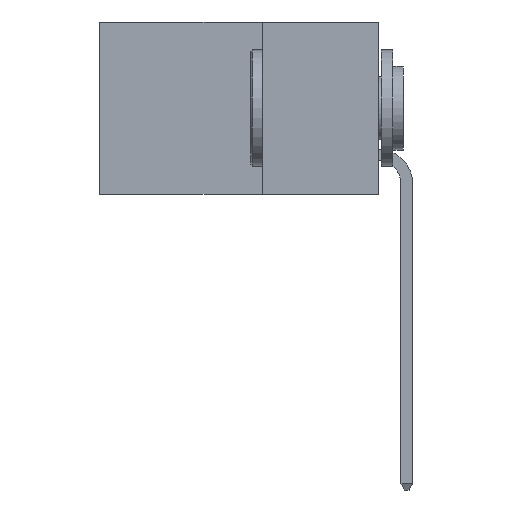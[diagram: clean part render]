
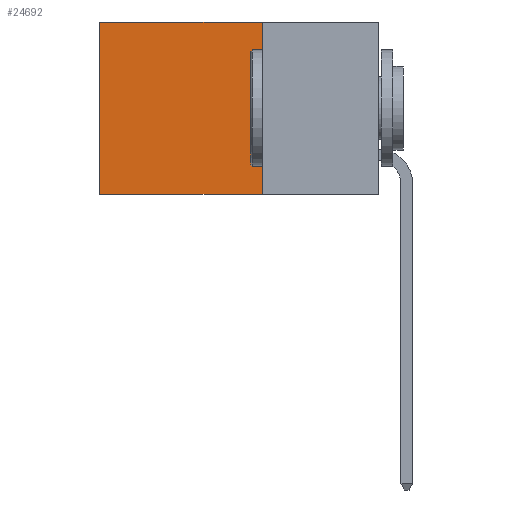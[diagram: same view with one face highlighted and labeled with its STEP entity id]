
A CAD part, left-side view. The second image highlights one B-rep face of the part: STEP entity #24692.
In plain terms, the highlighted planar face has unit normal (-1, 0, 0).
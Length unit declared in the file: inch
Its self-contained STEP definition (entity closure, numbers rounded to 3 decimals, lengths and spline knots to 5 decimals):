
#230 = EDGE_CURVE ( 'NONE', #22864, #7460, #1878, .T. ) ;
#1604 = DIRECTION ( 'NONE',  ( 0., 0., -1. ) ) ;
#1878 = LINE ( 'NONE', #25435, #7264 ) ;
#1979 = ORIENTED_EDGE ( 'NONE', *, *, #13694, .T. ) ;
#2709 = ORIENTED_EDGE ( 'NONE', *, *, #6600, .F. ) ;
#2841 = DIRECTION ( 'NONE',  ( 0., 1., 0. ) ) ;
#3092 = VERTEX_POINT ( 'NONE', #8693 ) ;
#3815 = CARTESIAN_POINT ( 'NONE',  ( 0.2615, 0.25, -0.37 ) ) ;
#4625 = LINE ( 'NONE', #17187, #9409 ) ;
#4657 = CARTESIAN_POINT ( 'NONE',  ( 0.2615, 0.25, -0.37 ) ) ;
#6600 = EDGE_CURVE ( 'NONE', #7460, #15725, #18814, .T. ) ;
#7002 = EDGE_CURVE ( 'NONE', #3092, #15725, #4625, .T. ) ;
#7264 = VECTOR ( 'NONE', #1604, 39.37008 ) ;
#7460 = VERTEX_POINT ( 'NONE', #4657 ) ;
#8693 = CARTESIAN_POINT ( 'NONE',  ( 0.2615, 0.6, 0. ) ) ;
#8945 = CARTESIAN_POINT ( 'NONE',  ( 0.2615, 0.25, 0. ) ) ;
#9215 = DIRECTION ( 'NONE',  ( 0., 0., -1. ) ) ;
#9409 = VECTOR ( 'NONE', #9215, 39.37008 ) ;
#10236 = DIRECTION ( 'NONE',  ( 1., 0., 0. ) ) ;
#12138 = CARTESIAN_POINT ( 'NONE',  ( 0.2615, 0.6, -0.37 ) ) ;
#12934 = LINE ( 'NONE', #8945, #22245 ) ;
#13522 = VECTOR ( 'NONE', #21881, 39.37008 ) ;
#13694 = EDGE_CURVE ( 'NONE', #22864, #3092, #12934, .T. ) ;
#14758 = PLANE ( 'NONE',  #21712 ) ;
#15725 = VERTEX_POINT ( 'NONE', #12138 ) ;
#15941 = EDGE_LOOP ( 'NONE', ( #25097, #2709, #22214, #1979 ) ) ;
#17187 = CARTESIAN_POINT ( 'NONE',  ( 0.2615, 0.6, -0.37 ) ) ;
#18814 = LINE ( 'NONE', #3815, #13522 ) ;
#18992 = CARTESIAN_POINT ( 'NONE',  ( 0.2615, 0.25, 0. ) ) ;
#21712 = AXIS2_PLACEMENT_3D ( 'NONE', #22138, #10236, #24152 ) ;
#21881 = DIRECTION ( 'NONE',  ( 0., 1., 0. ) ) ;
#22138 = CARTESIAN_POINT ( 'NONE',  ( 0.2615, 0.25, -0.37 ) ) ;
#22214 = ORIENTED_EDGE ( 'NONE', *, *, #230, .F. ) ;
#22245 = VECTOR ( 'NONE', #2841, 39.37008 ) ;
#22864 = VERTEX_POINT ( 'NONE', #18992 ) ;
#24152 = DIRECTION ( 'NONE',  ( 0., 0., -1. ) ) ;
#24525 = FACE_OUTER_BOUND ( 'NONE', #15941, .T. ) ;
#24692 = ADVANCED_FACE ( 'NONE', ( #24525 ), #14758, .F. ) ;
#25097 = ORIENTED_EDGE ( 'NONE', *, *, #7002, .T. ) ;
#25435 = CARTESIAN_POINT ( 'NONE',  ( 0.2615, 0.25, -0.37 ) ) ;
